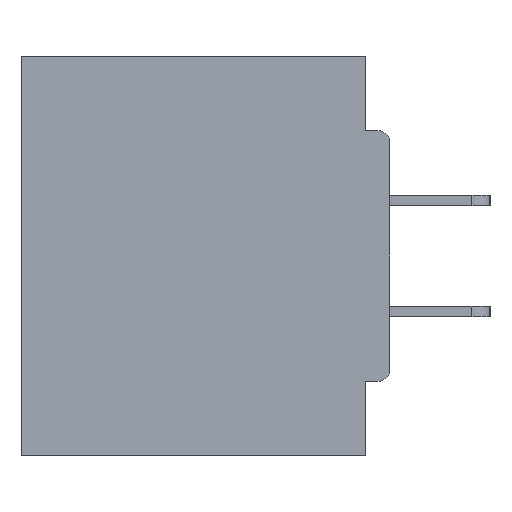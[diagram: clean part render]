
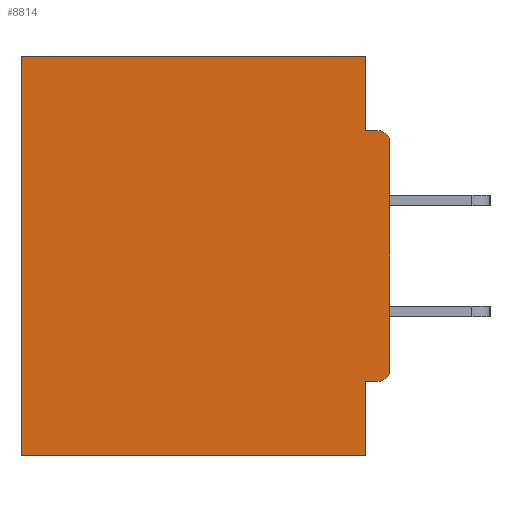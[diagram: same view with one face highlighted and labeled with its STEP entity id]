
A CAD part, left-side view. The second image highlights one B-rep face of the part: STEP entity #8814.
In plain terms, the highlighted planar face has unit normal (-1, 0, 0).
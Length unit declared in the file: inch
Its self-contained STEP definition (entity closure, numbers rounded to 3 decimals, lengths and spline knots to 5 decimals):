
#253 = EDGE_CURVE ( 'NONE', #11858, #18526, #25096, .T. ) ;
#366 = CARTESIAN_POINT ( 'NONE',  ( 0.298, 0.031, -0.4065 ) ) ;
#932 = VERTEX_POINT ( 'NONE', #16119 ) ;
#2153 = CARTESIAN_POINT ( 'NONE',  ( 0.298, 0.015, -0.4065 ) ) ;
#2373 = CARTESIAN_POINT ( 'NONE',  ( 0.298, 0., -0.3915 ) ) ;
#2719 = ORIENTED_EDGE ( 'NONE', *, *, #36301, .F. ) ;
#2880 = VERTEX_POINT ( 'NONE', #2373 ) ;
#3058 = VERTEX_POINT ( 'NONE', #31852 ) ;
#3507 = CARTESIAN_POINT ( 'NONE',  ( 0.298, 0., -0.0935 ) ) ;
#5389 = DIRECTION ( 'NONE',  ( 0., 0., -1. ) ) ;
#6639 = DIRECTION ( 'NONE',  ( 0., 0., -1. ) ) ;
#6717 = VECTOR ( 'NONE', #20274, 39.37008 ) ;
#6747 = CIRCLE ( 'NONE', #17758, 0.015 ) ;
#6967 = DIRECTION ( 'NONE',  ( -1., 0., 0. ) ) ;
#7335 = DIRECTION ( 'NONE',  ( 0., 0., -1. ) ) ;
#7419 = CARTESIAN_POINT ( 'NONE',  ( 0.298, 0.031, -0.5 ) ) ;
#8483 = VECTOR ( 'NONE', #15237, 39.37008 ) ;
#8814 = ADVANCED_FACE ( 'NONE', ( #15699 ), #29610, .F. ) ;
#9649 = CARTESIAN_POINT ( 'NONE',  ( 0.298, 0., 0. ) ) ;
#10886 = CARTESIAN_POINT ( 'NONE',  ( 0.298, 0., -0.4065 ) ) ;
#11282 = CARTESIAN_POINT ( 'NONE',  ( 0.298, 0.031, -0.5 ) ) ;
#11415 = CARTESIAN_POINT ( 'NONE',  ( 0.298, 0.46, 0. ) ) ;
#11643 = ORIENTED_EDGE ( 'NONE', *, *, #30944, .T. ) ;
#11744 = ORIENTED_EDGE ( 'NONE', *, *, #33597, .F. ) ;
#11858 = VERTEX_POINT ( 'NONE', #21861 ) ;
#11981 = DIRECTION ( 'NONE',  ( 0., -1., 0. ) ) ;
#12074 = DIRECTION ( 'NONE',  ( 0., 1., 0. ) ) ;
#12766 = LINE ( 'NONE', #3507, #35771 ) ;
#13073 = ORIENTED_EDGE ( 'NONE', *, *, #18140, .F. ) ;
#13447 = LINE ( 'NONE', #26619, #8483 ) ;
#13660 = ORIENTED_EDGE ( 'NONE', *, *, #31171, .F. ) ;
#14337 = CARTESIAN_POINT ( 'NONE',  ( 0.298, 0., -0.5 ) ) ;
#14884 = AXIS2_PLACEMENT_3D ( 'NONE', #32248, #26494, #6639 ) ;
#15048 = VECTOR ( 'NONE', #30382, 39.37008 ) ;
#15229 = CARTESIAN_POINT ( 'NONE',  ( 0.298, 0.015, -0.0935 ) ) ;
#15237 = DIRECTION ( 'NONE',  ( 0., 0., -1. ) ) ;
#15699 = FACE_OUTER_BOUND ( 'NONE', #19151, .T. ) ;
#16119 = CARTESIAN_POINT ( 'NONE',  ( 0.298, 0.031, -0.5 ) ) ;
#16423 = DIRECTION ( 'NONE',  ( 0., 1., 0. ) ) ;
#16438 = VECTOR ( 'NONE', #16423, 39.37008 ) ;
#16613 = CARTESIAN_POINT ( 'NONE',  ( 0.298, 0.015, -0.3915 ) ) ;
#17678 = ORIENTED_EDGE ( 'NONE', *, *, #33757, .F. ) ;
#17758 = AXIS2_PLACEMENT_3D ( 'NONE', #16613, #31098, #5389 ) ;
#18140 = EDGE_CURVE ( 'NONE', #20364, #25623, #34451, .T. ) ;
#18526 = VERTEX_POINT ( 'NONE', #15229 ) ;
#19151 = EDGE_LOOP ( 'NONE', ( #27750, #2719, #13073, #33361, #30188, #13660, #11744, #36817, #11643, #17678 ) ) ;
#20274 = DIRECTION ( 'NONE',  ( 0., 1., 0. ) ) ;
#20364 = VERTEX_POINT ( 'NONE', #22182 ) ;
#21473 = CARTESIAN_POINT ( 'NONE',  ( 0.298, 0.015, -0.1085 ) ) ;
#21861 = CARTESIAN_POINT ( 'NONE',  ( 0.298, 0., -0.1085 ) ) ;
#21867 = LINE ( 'NONE', #10886, #16438 ) ;
#22182 = CARTESIAN_POINT ( 'NONE',  ( 0.298, 0.031, 0. ) ) ;
#22931 = LINE ( 'NONE', #11282, #27887 ) ;
#23631 = VECTOR ( 'NONE', #12074, 39.37008 ) ;
#23882 = CARTESIAN_POINT ( 'NONE',  ( 0.298, 0.031, -0.0935 ) ) ;
#24516 = CARTESIAN_POINT ( 'NONE',  ( 0.298, 0.46, 0. ) ) ;
#24804 = LINE ( 'NONE', #14337, #6717 ) ;
#25096 = CIRCLE ( 'NONE', #30001, 0.015 ) ;
#25623 = VERTEX_POINT ( 'NONE', #23882 ) ;
#26272 = VECTOR ( 'NONE', #33166, 39.37008 ) ;
#26494 = DIRECTION ( 'NONE',  ( 1., 0., 0. ) ) ;
#26619 = CARTESIAN_POINT ( 'NONE',  ( 0.298, 0., 0. ) ) ;
#27750 = ORIENTED_EDGE ( 'NONE', *, *, #253, .T. ) ;
#27887 = VECTOR ( 'NONE', #34347, 39.37008 ) ;
#28110 = VERTEX_POINT ( 'NONE', #2153 ) ;
#28353 = VERTEX_POINT ( 'NONE', #366 ) ;
#29176 = EDGE_CURVE ( 'NONE', #20364, #33581, #34878, .T. ) ;
#29610 = PLANE ( 'NONE',  #14884 ) ;
#29844 = EDGE_CURVE ( 'NONE', #33581, #3058, #33891, .T. ) ;
#30001 = AXIS2_PLACEMENT_3D ( 'NONE', #21473, #6967, #7335 ) ;
#30188 = ORIENTED_EDGE ( 'NONE', *, *, #29844, .T. ) ;
#30382 = DIRECTION ( 'NONE',  ( 0., 0., -1. ) ) ;
#30944 = EDGE_CURVE ( 'NONE', #28110, #2880, #6747, .T. ) ;
#31098 = DIRECTION ( 'NONE',  ( -1., 0., 0. ) ) ;
#31171 = EDGE_CURVE ( 'NONE', #932, #3058, #24804, .T. ) ;
#31852 = CARTESIAN_POINT ( 'NONE',  ( 0.298, 0.46, -0.5 ) ) ;
#32248 = CARTESIAN_POINT ( 'NONE',  ( 0.298, 0., 0. ) ) ;
#33166 = DIRECTION ( 'NONE',  ( 0., 0., -1. ) ) ;
#33361 = ORIENTED_EDGE ( 'NONE', *, *, #29176, .T. ) ;
#33581 = VERTEX_POINT ( 'NONE', #11415 ) ;
#33597 = EDGE_CURVE ( 'NONE', #28353, #932, #22931, .T. ) ;
#33757 = EDGE_CURVE ( 'NONE', #11858, #2880, #13447, .T. ) ;
#33891 = LINE ( 'NONE', #24516, #26272 ) ;
#34347 = DIRECTION ( 'NONE',  ( 0., 0., -1. ) ) ;
#34451 = LINE ( 'NONE', #7419, #15048 ) ;
#34878 = LINE ( 'NONE', #9649, #23631 ) ;
#35287 = EDGE_CURVE ( 'NONE', #28110, #28353, #21867, .T. ) ;
#35771 = VECTOR ( 'NONE', #11981, 39.37008 ) ;
#36301 = EDGE_CURVE ( 'NONE', #25623, #18526, #12766, .T. ) ;
#36817 = ORIENTED_EDGE ( 'NONE', *, *, #35287, .F. ) ;
